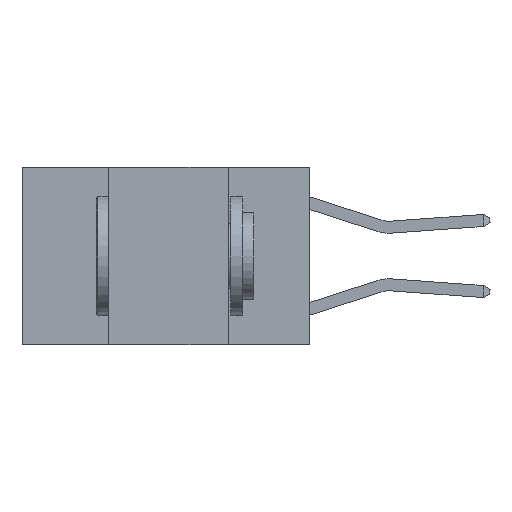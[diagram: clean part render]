
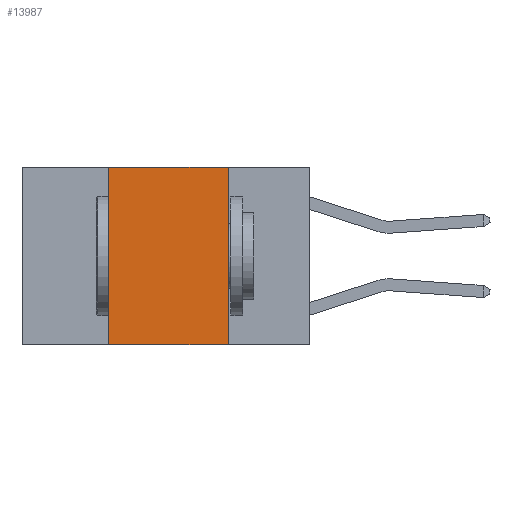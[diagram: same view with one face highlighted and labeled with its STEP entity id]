
A CAD part, left-side view. The second image highlights one B-rep face of the part: STEP entity #13987.
In plain terms, the highlighted planar face has unit normal (-1, 0, 0).
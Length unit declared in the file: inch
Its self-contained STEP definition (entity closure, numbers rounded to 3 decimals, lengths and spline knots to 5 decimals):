
#1621 = EDGE_CURVE ( 'NONE', #8095, #13061, #6720, .T. ) ;
#1624 = CARTESIAN_POINT ( 'NONE',  ( 0., 0.42, -0.37 ) ) ;
#1699 = PLANE ( 'NONE',  #3599 ) ;
#1759 = EDGE_LOOP ( 'NONE', ( #3193, #9227, #5209, #14299 ) ) ;
#2388 = EDGE_CURVE ( 'NONE', #13620, #13061, #14816, .T. ) ;
#2973 = CARTESIAN_POINT ( 'NONE',  ( 0., 0.17, -0.37 ) ) ;
#3020 = EDGE_CURVE ( 'NONE', #8095, #15670, #5693, .T. ) ;
#3193 = ORIENTED_EDGE ( 'NONE', *, *, #2388, .F. ) ;
#3211 = DIRECTION ( 'NONE',  ( 0., -1., 0. ) ) ;
#3583 = LINE ( 'NONE', #7077, #7354 ) ;
#3599 = AXIS2_PLACEMENT_3D ( 'NONE', #7792, #12625, #15267 ) ;
#4611 = CARTESIAN_POINT ( 'NONE',  ( 0., 0.17, 0. ) ) ;
#5179 = VECTOR ( 'NONE', #10536, 39.37008 ) ;
#5209 = ORIENTED_EDGE ( 'NONE', *, *, #3020, .F. ) ;
#5693 = LINE ( 'NONE', #15169, #5179 ) ;
#6720 = LINE ( 'NONE', #11651, #13572 ) ;
#6813 = FACE_OUTER_BOUND ( 'NONE', #1759, .T. ) ;
#7077 = CARTESIAN_POINT ( 'NONE',  ( 0., 0.6, 0. ) ) ;
#7354 = VECTOR ( 'NONE', #11933, 39.37008 ) ;
#7792 = CARTESIAN_POINT ( 'NONE',  ( 0., 0.6, 0. ) ) ;
#8095 = VERTEX_POINT ( 'NONE', #1624 ) ;
#8356 = VECTOR ( 'NONE', #8993, 39.37008 ) ;
#8993 = DIRECTION ( 'NONE',  ( 0., 0., -1. ) ) ;
#9227 = ORIENTED_EDGE ( 'NONE', *, *, #9826, .F. ) ;
#9826 = EDGE_CURVE ( 'NONE', #15670, #13620, #3583, .T. ) ;
#10536 = DIRECTION ( 'NONE',  ( 0., 0., 1. ) ) ;
#11651 = CARTESIAN_POINT ( 'NONE',  ( 0., 0.6, -0.37 ) ) ;
#11933 = DIRECTION ( 'NONE',  ( 0., -1., 0. ) ) ;
#12625 = DIRECTION ( 'NONE',  ( 1., 0., 0. ) ) ;
#13061 = VERTEX_POINT ( 'NONE', #2973 ) ;
#13572 = VECTOR ( 'NONE', #3211, 39.37008 ) ;
#13620 = VERTEX_POINT ( 'NONE', #4611 ) ;
#13728 = CARTESIAN_POINT ( 'NONE',  ( 0., 0.42, 0. ) ) ;
#13901 = CARTESIAN_POINT ( 'NONE',  ( 0., 0.17, 0. ) ) ;
#13987 = ADVANCED_FACE ( 'NONE', ( #6813 ), #1699, .F. ) ;
#14299 = ORIENTED_EDGE ( 'NONE', *, *, #1621, .T. ) ;
#14816 = LINE ( 'NONE', #13901, #8356 ) ;
#15169 = CARTESIAN_POINT ( 'NONE',  ( 0., 0.42, 0. ) ) ;
#15267 = DIRECTION ( 'NONE',  ( 0., 0., -1. ) ) ;
#15670 = VERTEX_POINT ( 'NONE', #13728 ) ;
